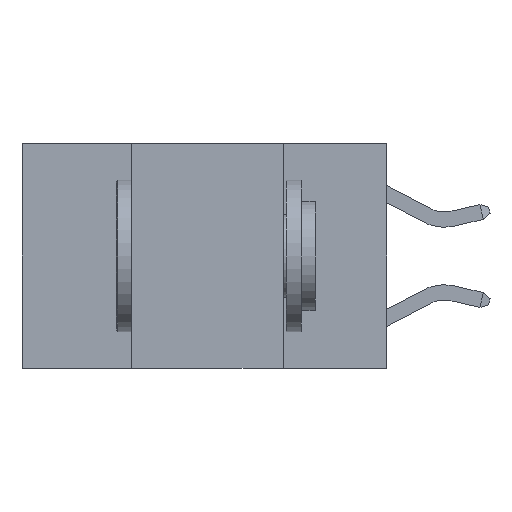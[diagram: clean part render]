
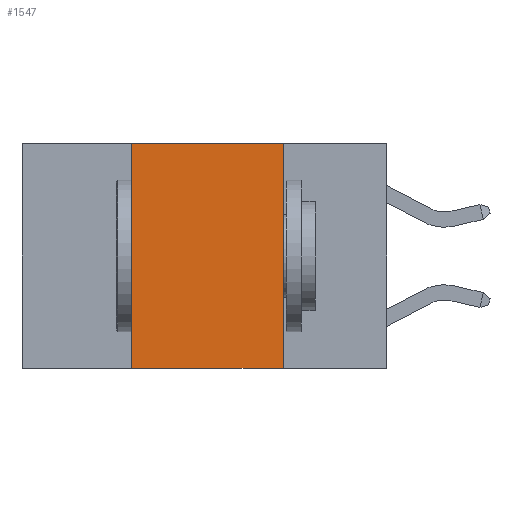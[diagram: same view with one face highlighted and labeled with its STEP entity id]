
A CAD part, left-side view. The second image highlights one B-rep face of the part: STEP entity #1547.
In plain terms, the highlighted planar face has unit normal (-1, 0, 0).
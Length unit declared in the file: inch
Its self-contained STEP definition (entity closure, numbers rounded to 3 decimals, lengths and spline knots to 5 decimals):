
#130 = CARTESIAN_POINT ( 'NONE',  ( 0., 0.17, 0. ) ) ;
#309 = VERTEX_POINT ( 'NONE', #5299 ) ;
#325 = DIRECTION ( 'NONE',  ( 0., -1., 0. ) ) ;
#512 = CARTESIAN_POINT ( 'NONE',  ( 0., 0.6, -0.37 ) ) ;
#534 = ORIENTED_EDGE ( 'NONE', *, *, #8572, .T. ) ;
#1064 = VECTOR ( 'NONE', #5879, 39.37008 ) ;
#1236 = VECTOR ( 'NONE', #325, 39.37008 ) ;
#1547 = ADVANCED_FACE ( 'NONE', ( #6059 ), #6309, .F. ) ;
#2001 = EDGE_CURVE ( 'NONE', #10473, #3524, #3360, .T. ) ;
#2199 = CARTESIAN_POINT ( 'NONE',  ( 0., 0.6, 0. ) ) ;
#2247 = DIRECTION ( 'NONE',  ( 0., 0., 1. ) ) ;
#2373 = CARTESIAN_POINT ( 'NONE',  ( 0., 0.42, 0. ) ) ;
#2386 = DIRECTION ( 'NONE',  ( 1., 0., 0. ) ) ;
#2570 = DIRECTION ( 'NONE',  ( 0., -1., 0. ) ) ;
#2675 = AXIS2_PLACEMENT_3D ( 'NONE', #10941, #2386, #7163 ) ;
#3360 = LINE ( 'NONE', #2373, #8816 ) ;
#3524 = VERTEX_POINT ( 'NONE', #3735 ) ;
#3735 = CARTESIAN_POINT ( 'NONE',  ( 0., 0.42, 0. ) ) ;
#4383 = CARTESIAN_POINT ( 'NONE',  ( 0., 0.17, -0.37 ) ) ;
#5100 = ORIENTED_EDGE ( 'NONE', *, *, #12186, .F. ) ;
#5299 = CARTESIAN_POINT ( 'NONE',  ( 0., 0.17, 0. ) ) ;
#5531 = EDGE_LOOP ( 'NONE', ( #8407, #5100, #8224, #534 ) ) ;
#5825 = EDGE_CURVE ( 'NONE', #309, #8259, #8653, .T. ) ;
#5879 = DIRECTION ( 'NONE',  ( 0., 0., -1. ) ) ;
#6059 = FACE_OUTER_BOUND ( 'NONE', #5531, .T. ) ;
#6309 = PLANE ( 'NONE',  #2675 ) ;
#7163 = DIRECTION ( 'NONE',  ( 0., 0., -1. ) ) ;
#7817 = VECTOR ( 'NONE', #2570, 39.37008 ) ;
#7975 = CARTESIAN_POINT ( 'NONE',  ( 0., 0.42, -0.37 ) ) ;
#8224 = ORIENTED_EDGE ( 'NONE', *, *, #2001, .F. ) ;
#8259 = VERTEX_POINT ( 'NONE', #4383 ) ;
#8407 = ORIENTED_EDGE ( 'NONE', *, *, #5825, .F. ) ;
#8572 = EDGE_CURVE ( 'NONE', #10473, #8259, #9088, .T. ) ;
#8653 = LINE ( 'NONE', #130, #1064 ) ;
#8816 = VECTOR ( 'NONE', #2247, 39.37008 ) ;
#9088 = LINE ( 'NONE', #512, #7817 ) ;
#9890 = LINE ( 'NONE', #2199, #1236 ) ;
#10473 = VERTEX_POINT ( 'NONE', #7975 ) ;
#10941 = CARTESIAN_POINT ( 'NONE',  ( 0., 0.6, 0. ) ) ;
#12186 = EDGE_CURVE ( 'NONE', #3524, #309, #9890, .T. ) ;
